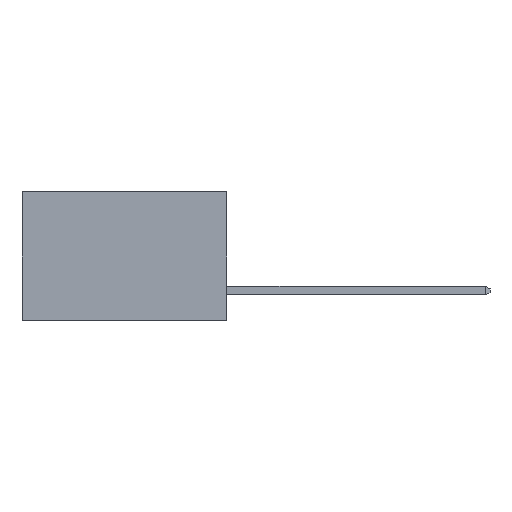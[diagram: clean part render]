
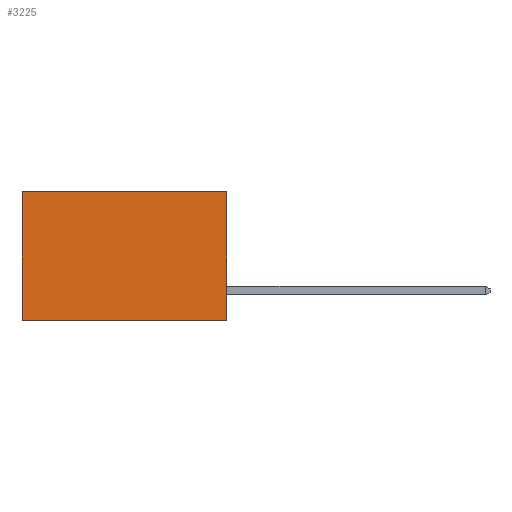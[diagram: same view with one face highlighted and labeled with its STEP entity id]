
A CAD part, left-side view. The second image highlights one B-rep face of the part: STEP entity #3225.
In plain terms, the highlighted planar face has unit normal (-1, 0, 0).
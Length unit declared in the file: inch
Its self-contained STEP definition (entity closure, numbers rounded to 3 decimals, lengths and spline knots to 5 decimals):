
#240 = CARTESIAN_POINT ( 'NONE',  ( 0.277, 0.59, -0.37 ) ) ;
#273 = DIRECTION ( 'NONE',  ( 0., 0., -1. ) ) ;
#505 = ORIENTED_EDGE ( 'NONE', *, *, #2143, .F. ) ;
#2086 = VERTEX_POINT ( 'NONE', #5091 ) ;
#2143 = EDGE_CURVE ( 'NONE', #4136, #6507, #6062, .T. ) ;
#2197 = CARTESIAN_POINT ( 'NONE',  ( 0.277, 0., -0.37 ) ) ;
#2289 = EDGE_CURVE ( 'NONE', #2086, #4136, #3482, .T. ) ;
#2407 = CARTESIAN_POINT ( 'NONE',  ( 0.277, 0.59, 0. ) ) ;
#3180 = ORIENTED_EDGE ( 'NONE', *, *, #6755, .T. ) ;
#3203 = CARTESIAN_POINT ( 'NONE',  ( 0.277, 0., -0.37 ) ) ;
#3225 = ADVANCED_FACE ( 'NONE', ( #7215 ), #6350, .F. ) ;
#3479 = VECTOR ( 'NONE', #273, 39.37008 ) ;
#3482 = LINE ( 'NONE', #7750, #6319 ) ;
#4136 = VERTEX_POINT ( 'NONE', #2197 ) ;
#4509 = LINE ( 'NONE', #6778, #5843 ) ;
#4546 = CARTESIAN_POINT ( 'NONE',  ( 0.277, 0.59, -0.37 ) ) ;
#4610 = ORIENTED_EDGE ( 'NONE', *, *, #2289, .F. ) ;
#4909 = VECTOR ( 'NONE', #7447, 39.37008 ) ;
#5091 = CARTESIAN_POINT ( 'NONE',  ( 0.277, 0., 0. ) ) ;
#5709 = EDGE_CURVE ( 'NONE', #2086, #6130, #4509, .T. ) ;
#5772 = AXIS2_PLACEMENT_3D ( 'NONE', #6388, #6158, #6067 ) ;
#5843 = VECTOR ( 'NONE', #6546, 39.37008 ) ;
#5990 = EDGE_LOOP ( 'NONE', ( #3180, #505, #4610, #6616 ) ) ;
#6062 = LINE ( 'NONE', #3203, #4909 ) ;
#6067 = DIRECTION ( 'NONE',  ( 0., 0., -1. ) ) ;
#6130 = VERTEX_POINT ( 'NONE', #2407 ) ;
#6158 = DIRECTION ( 'NONE',  ( 1., 0., 0. ) ) ;
#6319 = VECTOR ( 'NONE', #7032, 39.37008 ) ;
#6350 = PLANE ( 'NONE',  #5772 ) ;
#6388 = CARTESIAN_POINT ( 'NONE',  ( 0.277, 0., -0.37 ) ) ;
#6507 = VERTEX_POINT ( 'NONE', #4546 ) ;
#6517 = LINE ( 'NONE', #240, #3479 ) ;
#6546 = DIRECTION ( 'NONE',  ( 0., 1., 0. ) ) ;
#6616 = ORIENTED_EDGE ( 'NONE', *, *, #5709, .T. ) ;
#6755 = EDGE_CURVE ( 'NONE', #6130, #6507, #6517, .T. ) ;
#6778 = CARTESIAN_POINT ( 'NONE',  ( 0.277, 0., 0. ) ) ;
#7032 = DIRECTION ( 'NONE',  ( 0., 0., -1. ) ) ;
#7215 = FACE_OUTER_BOUND ( 'NONE', #5990, .T. ) ;
#7447 = DIRECTION ( 'NONE',  ( 0., 1., 0. ) ) ;
#7750 = CARTESIAN_POINT ( 'NONE',  ( 0.277, 0., -0.37 ) ) ;
